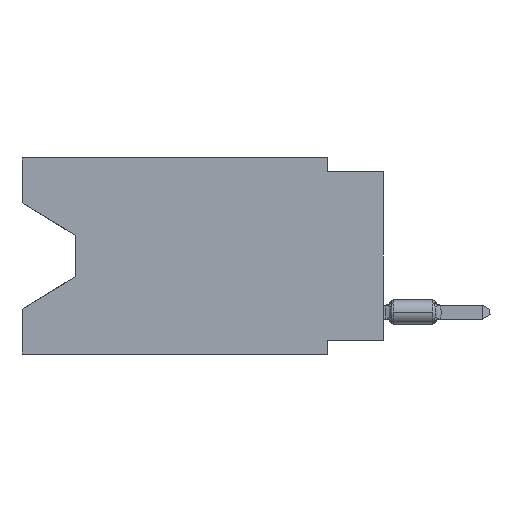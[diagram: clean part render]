
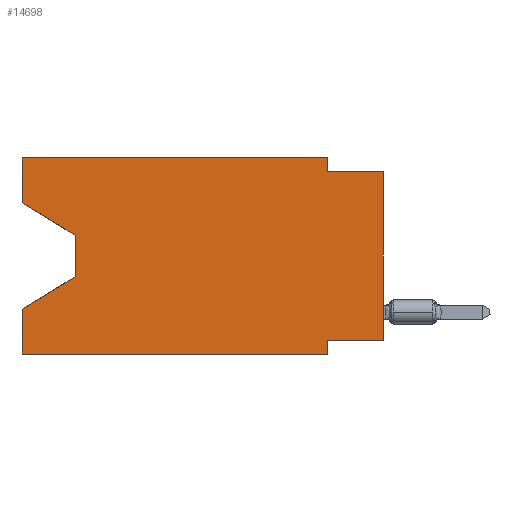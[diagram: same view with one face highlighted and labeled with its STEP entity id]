
A CAD part, left-side view. The second image highlights one B-rep face of the part: STEP entity #14698.
In plain terms, the highlighted planar face has unit normal (-1, 0, 0).
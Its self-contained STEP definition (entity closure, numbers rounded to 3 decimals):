
#648 = VECTOR ( 'NONE', #91756, 1000. ) ;
#2058 = DIRECTION ( 'NONE',  ( 0., 0., -1. ) ) ;
#2385 = EDGE_CURVE ( 'NONE', #28299, #42126, #56953, .T. ) ;
#8600 = CARTESIAN_POINT ( 'NONE',  ( 0., 13.97, -3.505 ) ) ;
#8964 = ORIENTED_EDGE ( 'NONE', *, *, #68850, .F. ) ;
#9992 = AXIS2_PLACEMENT_3D ( 'NONE', #54796, #83189, #19399 ) ;
#10651 = ORIENTED_EDGE ( 'NONE', *, *, #44562, .F. ) ;
#10855 = VERTEX_POINT ( 'NONE', #53171 ) ;
#11237 = DIRECTION ( 'NONE',  ( 0., 0., 1. ) ) ;
#11346 = EDGE_CURVE ( 'NONE', #17226, #91045, #43763, .T. ) ;
#12849 = VECTOR ( 'NONE', #82261, 1000. ) ;
#14578 = CARTESIAN_POINT ( 'NONE',  ( 0., 0., -0.635 ) ) ;
#14698 = ADVANCED_FACE ( 'NONE', ( #48735 ), #75277, .F. ) ;
#14963 = CARTESIAN_POINT ( 'NONE',  ( 0., 0., -8.255 ) ) ;
#15485 = DIRECTION ( 'NONE',  ( 0., -1., 0. ) ) ;
#16462 = EDGE_CURVE ( 'NONE', #67319, #17226, #25201, .T. ) ;
#17107 = EDGE_CURVE ( 'NONE', #41358, #90310, #33918, .T. ) ;
#17226 = VERTEX_POINT ( 'NONE', #55807 ) ;
#18589 = CARTESIAN_POINT ( 'NONE',  ( 0., 2.54, -8.89 ) ) ;
#19131 = CARTESIAN_POINT ( 'NONE',  ( 0., 2.54, -0.635 ) ) ;
#19399 = DIRECTION ( 'NONE',  ( 0., 0., -1. ) ) ;
#20084 = VECTOR ( 'NONE', #30391, 1000. ) ;
#23025 = DIRECTION ( 'NONE',  ( 0., 0., -1. ) ) ;
#23228 = EDGE_CURVE ( 'NONE', #10855, #90310, #79822, .T. ) ;
#23589 = CARTESIAN_POINT ( 'NONE',  ( 0., 16.383, -2.038 ) ) ;
#24155 = ORIENTED_EDGE ( 'NONE', *, *, #16462, .T. ) ;
#24613 = VECTOR ( 'NONE', #83970, 1000. ) ;
#24726 = ORIENTED_EDGE ( 'NONE', *, *, #62645, .F. ) ;
#25144 = ORIENTED_EDGE ( 'NONE', *, *, #91363, .F. ) ;
#25201 = LINE ( 'NONE', #8600, #60955 ) ;
#25917 = CARTESIAN_POINT ( 'NONE',  ( 0., 16.383, -2.038 ) ) ;
#28299 = VERTEX_POINT ( 'NONE', #19131 ) ;
#30391 = DIRECTION ( 'NONE',  ( 0., 0., 1. ) ) ;
#33918 = LINE ( 'NONE', #34372, #50652 ) ;
#34372 = CARTESIAN_POINT ( 'NONE',  ( 0., 16.383, -8.89 ) ) ;
#35709 = EDGE_LOOP ( 'NONE', ( #61192, #24155, #71729, #24726, #36572, #82674, #10651, #89707, #55026, #8964, #47519, #25144 ) ) ;
#35861 = CARTESIAN_POINT ( 'NONE',  ( 0., 13.97, -5.385 ) ) ;
#36572 = ORIENTED_EDGE ( 'NONE', *, *, #17107, .T. ) ;
#37089 = LINE ( 'NONE', #72014, #45125 ) ;
#37382 = LINE ( 'NONE', #65772, #20084 ) ;
#37648 = VECTOR ( 'NONE', #2058, 1000. ) ;
#38105 = CARTESIAN_POINT ( 'NONE',  ( 0., 16.383, 0. ) ) ;
#40422 = VECTOR ( 'NONE', #15485, 1000. ) ;
#40748 = CARTESIAN_POINT ( 'NONE',  ( 0., 0., -0.635 ) ) ;
#40964 = CARTESIAN_POINT ( 'NONE',  ( 0., 16.383, -8.89 ) ) ;
#41358 = VERTEX_POINT ( 'NONE', #40964 ) ;
#41703 = LINE ( 'NONE', #71012, #43209 ) ;
#42126 = VERTEX_POINT ( 'NONE', #40748 ) ;
#43209 = VECTOR ( 'NONE', #70087, 1000. ) ;
#43671 = LINE ( 'NONE', #25917, #12849 ) ;
#43763 = LINE ( 'NONE', #35861, #648 ) ;
#44562 = EDGE_CURVE ( 'NONE', #66681, #10855, #37089, .T. ) ;
#44606 = VERTEX_POINT ( 'NONE', #23589 ) ;
#45125 = VECTOR ( 'NONE', #88287, 1000. ) ;
#47519 = ORIENTED_EDGE ( 'NONE', *, *, #64644, .F. ) ;
#48735 = FACE_OUTER_BOUND ( 'NONE', #35709, .T. ) ;
#49307 = LINE ( 'NONE', #57193, #50149 ) ;
#50149 = VECTOR ( 'NONE', #55383, 1000. ) ;
#50652 = VECTOR ( 'NONE', #62326, 1000. ) ;
#51867 = CARTESIAN_POINT ( 'NONE',  ( 0., 13.97, -3.505 ) ) ;
#53171 = CARTESIAN_POINT ( 'NONE',  ( 0., 2.54, -8.255 ) ) ;
#54796 = CARTESIAN_POINT ( 'NONE',  ( 0., 16.383, 0. ) ) ;
#55026 = ORIENTED_EDGE ( 'NONE', *, *, #2385, .F. ) ;
#55383 = DIRECTION ( 'NONE',  ( 0., -1., 0. ) ) ;
#55585 = CARTESIAN_POINT ( 'NONE',  ( 0., 16.383, 0. ) ) ;
#55807 = CARTESIAN_POINT ( 'NONE',  ( 0., 13.97, -5.385 ) ) ;
#56953 = LINE ( 'NONE', #14578, #40422 ) ;
#57193 = CARTESIAN_POINT ( 'NONE',  ( 0., 16.383, 0. ) ) ;
#57742 = VECTOR ( 'NONE', #11237, 1000. ) ;
#60955 = VECTOR ( 'NONE', #23025, 1000. ) ;
#61192 = ORIENTED_EDGE ( 'NONE', *, *, #63599, .T. ) ;
#61982 = CARTESIAN_POINT ( 'NONE',  ( 0., 0., 0. ) ) ;
#62130 = CARTESIAN_POINT ( 'NONE',  ( 0., 16.383, -6.852 ) ) ;
#62326 = DIRECTION ( 'NONE',  ( 0., -1., 0. ) ) ;
#62645 = EDGE_CURVE ( 'NONE', #41358, #91045, #64826, .T. ) ;
#63599 = EDGE_CURVE ( 'NONE', #44606, #67319, #43671, .T. ) ;
#64644 = EDGE_CURVE ( 'NONE', #77463, #80583, #49307, .T. ) ;
#64826 = LINE ( 'NONE', #55585, #24613 ) ;
#65772 = CARTESIAN_POINT ( 'NONE',  ( 0., 16.383, 0. ) ) ;
#66681 = VERTEX_POINT ( 'NONE', #14963 ) ;
#67319 = VERTEX_POINT ( 'NONE', #51867 ) ;
#68850 = EDGE_CURVE ( 'NONE', #80583, #28299, #41703, .T. ) ;
#70087 = DIRECTION ( 'NONE',  ( 0., 0., -1. ) ) ;
#71012 = CARTESIAN_POINT ( 'NONE',  ( 0., 2.54, 0. ) ) ;
#71729 = ORIENTED_EDGE ( 'NONE', *, *, #11346, .T. ) ;
#72014 = CARTESIAN_POINT ( 'NONE',  ( 0., 0., -8.255 ) ) ;
#72363 = CARTESIAN_POINT ( 'NONE',  ( 0., 2.54, -8.89 ) ) ;
#75277 = PLANE ( 'NONE',  #9992 ) ;
#77463 = VERTEX_POINT ( 'NONE', #38105 ) ;
#79822 = LINE ( 'NONE', #72363, #37648 ) ;
#80583 = VERTEX_POINT ( 'NONE', #86417 ) ;
#82261 = DIRECTION ( 'NONE',  ( 0., -0.855, -0.519 ) ) ;
#82292 = EDGE_CURVE ( 'NONE', #66681, #42126, #82943, .T. ) ;
#82674 = ORIENTED_EDGE ( 'NONE', *, *, #23228, .F. ) ;
#82943 = LINE ( 'NONE', #61982, #57742 ) ;
#83189 = DIRECTION ( 'NONE',  ( 1., 0., 0. ) ) ;
#83970 = DIRECTION ( 'NONE',  ( 0., 0., 1. ) ) ;
#86417 = CARTESIAN_POINT ( 'NONE',  ( 0., 2.54, 0. ) ) ;
#88287 = DIRECTION ( 'NONE',  ( 0., 1., 0. ) ) ;
#89707 = ORIENTED_EDGE ( 'NONE', *, *, #82292, .T. ) ;
#90310 = VERTEX_POINT ( 'NONE', #18589 ) ;
#91045 = VERTEX_POINT ( 'NONE', #62130 ) ;
#91363 = EDGE_CURVE ( 'NONE', #44606, #77463, #37382, .T. ) ;
#91756 = DIRECTION ( 'NONE',  ( 0., 0.855, -0.519 ) ) ;
